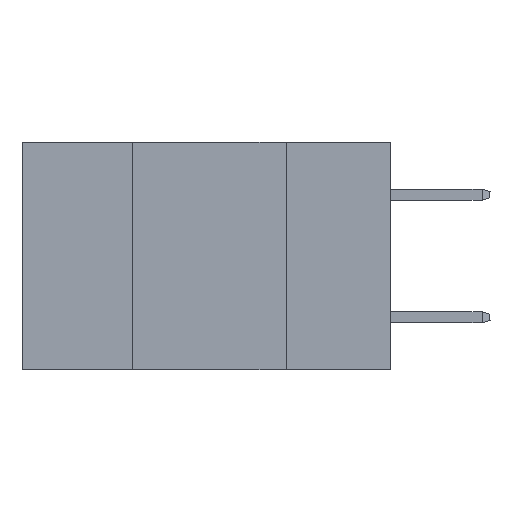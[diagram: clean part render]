
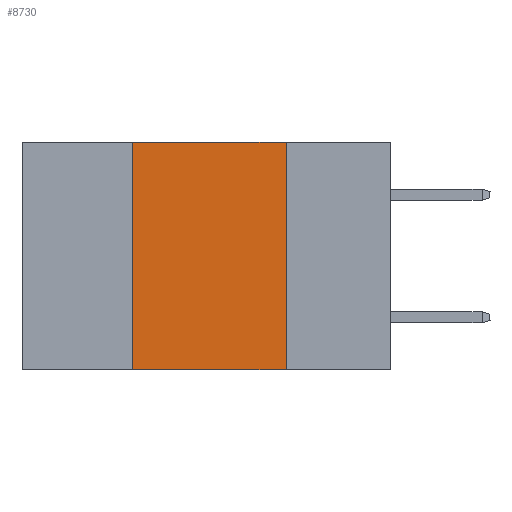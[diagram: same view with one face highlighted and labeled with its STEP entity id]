
A CAD part, left-side view. The second image highlights one B-rep face of the part: STEP entity #8730.
In plain terms, the highlighted planar face has unit normal (-1, 0, 0).
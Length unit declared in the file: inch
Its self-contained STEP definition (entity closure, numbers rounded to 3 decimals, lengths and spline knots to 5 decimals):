
#380 = DIRECTION ( 'NONE',  ( 1., 0., 0. ) ) ;
#421 = EDGE_CURVE ( 'NONE', #6355, #7127, #9264, .T. ) ;
#1327 = LINE ( 'NONE', #6553, #9486 ) ;
#2248 = CARTESIAN_POINT ( 'NONE',  ( 0., 0.42, 0. ) ) ;
#2777 = VERTEX_POINT ( 'NONE', #7097 ) ;
#3007 = VECTOR ( 'NONE', #7942, 39.37008 ) ;
#3091 = ORIENTED_EDGE ( 'NONE', *, *, #7297, .F. ) ;
#3263 = CARTESIAN_POINT ( 'NONE',  ( 0., 0.6, -0.37 ) ) ;
#3375 = AXIS2_PLACEMENT_3D ( 'NONE', #4896, #380, #7925 ) ;
#3607 = EDGE_CURVE ( 'NONE', #2777, #7590, #1327, .T. ) ;
#4085 = DIRECTION ( 'NONE',  ( 0., -1., 0. ) ) ;
#4565 = DIRECTION ( 'NONE',  ( 0., 0., 1. ) ) ;
#4629 = CARTESIAN_POINT ( 'NONE',  ( 0., 0.42, -0.37 ) ) ;
#4896 = CARTESIAN_POINT ( 'NONE',  ( 0., 0.6, 0. ) ) ;
#5045 = LINE ( 'NONE', #3263, #3007 ) ;
#5347 = ORIENTED_EDGE ( 'NONE', *, *, #6782, .T. ) ;
#5933 = CARTESIAN_POINT ( 'NONE',  ( 0., 0.17, -0.37 ) ) ;
#5976 = ORIENTED_EDGE ( 'NONE', *, *, #421, .F. ) ;
#6355 = VERTEX_POINT ( 'NONE', #4629 ) ;
#6457 = LINE ( 'NONE', #7076, #9408 ) ;
#6553 = CARTESIAN_POINT ( 'NONE',  ( 0., 0.17, 0. ) ) ;
#6671 = VECTOR ( 'NONE', #4565, 39.37008 ) ;
#6782 = EDGE_CURVE ( 'NONE', #6355, #7590, #5045, .T. ) ;
#6825 = ORIENTED_EDGE ( 'NONE', *, *, #3607, .F. ) ;
#7007 = PLANE ( 'NONE',  #3375 ) ;
#7076 = CARTESIAN_POINT ( 'NONE',  ( 0., 0.6, 0. ) ) ;
#7097 = CARTESIAN_POINT ( 'NONE',  ( 0., 0.17, 0. ) ) ;
#7127 = VERTEX_POINT ( 'NONE', #8287 ) ;
#7297 = EDGE_CURVE ( 'NONE', #7127, #2777, #6457, .T. ) ;
#7590 = VERTEX_POINT ( 'NONE', #5933 ) ;
#7925 = DIRECTION ( 'NONE',  ( 0., 0., -1. ) ) ;
#7942 = DIRECTION ( 'NONE',  ( 0., -1., 0. ) ) ;
#8078 = DIRECTION ( 'NONE',  ( 0., 0., -1. ) ) ;
#8138 = FACE_OUTER_BOUND ( 'NONE', #8897, .T. ) ;
#8287 = CARTESIAN_POINT ( 'NONE',  ( 0., 0.42, 0. ) ) ;
#8730 = ADVANCED_FACE ( 'NONE', ( #8138 ), #7007, .F. ) ;
#8897 = EDGE_LOOP ( 'NONE', ( #6825, #3091, #5976, #5347 ) ) ;
#9264 = LINE ( 'NONE', #2248, #6671 ) ;
#9408 = VECTOR ( 'NONE', #4085, 39.37008 ) ;
#9486 = VECTOR ( 'NONE', #8078, 39.37008 ) ;
